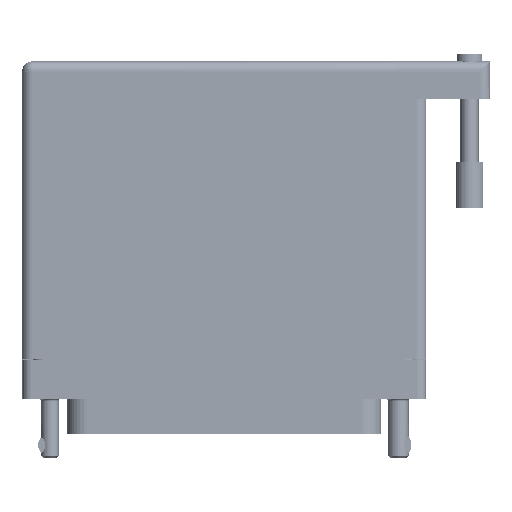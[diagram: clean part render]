
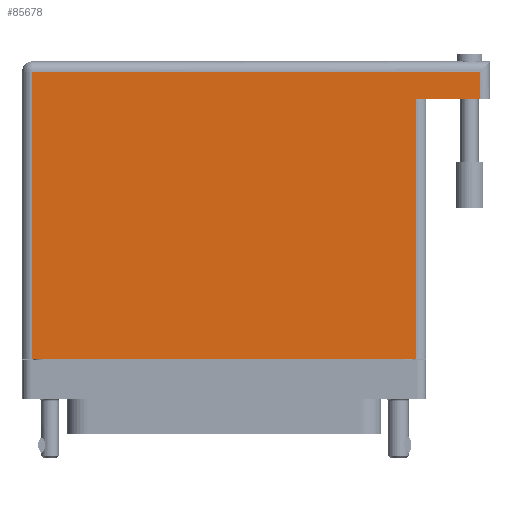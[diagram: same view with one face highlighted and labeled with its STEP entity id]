
A CAD part, front view. The second image highlights one B-rep face of the part: STEP entity #85678.
In plain terms, the highlighted face is planar.
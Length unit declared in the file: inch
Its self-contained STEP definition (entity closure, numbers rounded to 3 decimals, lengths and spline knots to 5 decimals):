
#3902 = CARTESIAN_POINT ( 'NONE',  ( -1.3075, -0.1, 0.765 ) ) ;
#6151 = VERTEX_POINT ( 'NONE', #31130 ) ;
#9101 = ORIENTED_EDGE ( 'NONE', *, *, #72023, .T. ) ;
#9516 = CARTESIAN_POINT ( 'NONE',  ( -1.3775, 1.93, 0.765 ) ) ;
#9622 = VECTOR ( 'NONE', #40105, 39.37008 ) ;
#10219 = CARTESIAN_POINT ( 'NONE',  ( -1.3075, 1.86, 0.765 ) ) ;
#11051 = DIRECTION ( 'NONE',  ( -1., 0., 0. ) ) ;
#11060 = EDGE_CURVE ( 'NONE', #6151, #46812, #71815, .T. ) ;
#12350 = EDGE_CURVE ( 'NONE', #63663, #6151, #27932, .T. ) ;
#12600 = VECTOR ( 'NONE', #58666, 39.37008 ) ;
#15282 = EDGE_CURVE ( 'NONE', #46812, #44386, #60100, .T. ) ;
#20141 = CARTESIAN_POINT ( 'NONE',  ( 1.7425, 1.93, 0.765 ) ) ;
#23163 = ORIENTED_EDGE ( 'NONE', *, *, #15282, .T. ) ;
#25688 = VERTEX_POINT ( 'NONE', #58007 ) ;
#27749 = VERTEX_POINT ( 'NONE', #46217 ) ;
#27914 = LINE ( 'NONE', #51870, #12600 ) ;
#27932 = LINE ( 'NONE', #20141, #72833 ) ;
#31130 = CARTESIAN_POINT ( 'NONE',  ( 1.7425, 1.86, 0.765 ) ) ;
#34433 = CARTESIAN_POINT ( 'NONE',  ( 1.7425, 1.674, 0.765 ) ) ;
#36376 = DIRECTION ( 'NONE',  ( 1., 0., 0. ) ) ;
#36627 = VECTOR ( 'NONE', #36376, 39.37008 ) ;
#40105 = DIRECTION ( 'NONE',  ( -1., 0., 0. ) ) ;
#42818 = DIRECTION ( 'NONE',  ( 0., 0., -1. ) ) ;
#44087 = DIRECTION ( 'NONE',  ( 0., 1., 0. ) ) ;
#44386 = VERTEX_POINT ( 'NONE', #70392 ) ;
#44701 = CARTESIAN_POINT ( 'NONE',  ( -1.3775, -0.1, 0.765 ) ) ;
#46217 = CARTESIAN_POINT ( 'NONE',  ( 1.3075, 1.674, 0.765 ) ) ;
#46812 = VERTEX_POINT ( 'NONE', #10219 ) ;
#46900 = ORIENTED_EDGE ( 'NONE', *, *, #11060, .T. ) ;
#51870 = CARTESIAN_POINT ( 'NONE',  ( 1.3075, 1.674, 0.765 ) ) ;
#58007 = CARTESIAN_POINT ( 'NONE',  ( 1.3075, -0.1, 0.765 ) ) ;
#58666 = DIRECTION ( 'NONE',  ( 0., 1., 0. ) ) ;
#60100 = LINE ( 'NONE', #3902, #66340 ) ;
#61083 = ORIENTED_EDGE ( 'NONE', *, *, #12350, .T. ) ;
#63663 = VERTEX_POINT ( 'NONE', #34433 ) ;
#66340 = VECTOR ( 'NONE', #76194, 39.37008 ) ;
#70392 = CARTESIAN_POINT ( 'NONE',  ( -1.3075, -0.1, 0.765 ) ) ;
#71071 = VECTOR ( 'NONE', #11051, 39.37008 ) ;
#71815 = LINE ( 'NONE', #80660, #9622 ) ;
#72023 = EDGE_CURVE ( 'NONE', #25688, #27749, #27914, .T. ) ;
#72833 = VECTOR ( 'NONE', #44087, 39.37008 ) ;
#74027 = LINE ( 'NONE', #75550, #71071 ) ;
#74183 = EDGE_CURVE ( 'NONE', #63663, #27749, #74027, .T. ) ;
#74518 = DIRECTION ( 'NONE',  ( -1., 0., 0. ) ) ;
#75550 = CARTESIAN_POINT ( 'NONE',  ( 1.8125, 1.674, 0.765 ) ) ;
#76194 = DIRECTION ( 'NONE',  ( 0., -1., 0. ) ) ;
#80660 = CARTESIAN_POINT ( 'NONE',  ( -1.3775, 1.86, 0.765 ) ) ;
#80829 = FACE_OUTER_BOUND ( 'NONE', #86312, .T. ) ;
#85678 = ADVANCED_FACE ( 'NONE', ( #80829 ), #88639, .F. ) ;
#86312 = EDGE_LOOP ( 'NONE', ( #93378, #9101, #99841, #61083, #46900, #23163 ) ) ;
#88639 = PLANE ( 'NONE',  #94498 ) ;
#93378 = ORIENTED_EDGE ( 'NONE', *, *, #100997, .T. ) ;
#94498 = AXIS2_PLACEMENT_3D ( 'NONE', #9516, #42818, #74518 ) ;
#98817 = LINE ( 'NONE', #44701, #36627 ) ;
#99841 = ORIENTED_EDGE ( 'NONE', *, *, #74183, .F. ) ;
#100997 = EDGE_CURVE ( 'NONE', #44386, #25688, #98817, .T. ) ;
